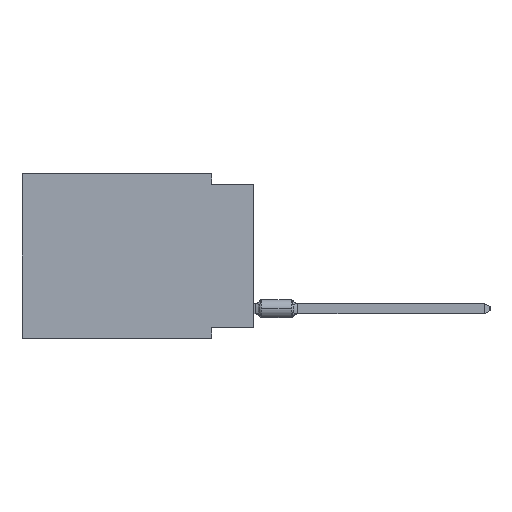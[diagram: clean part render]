
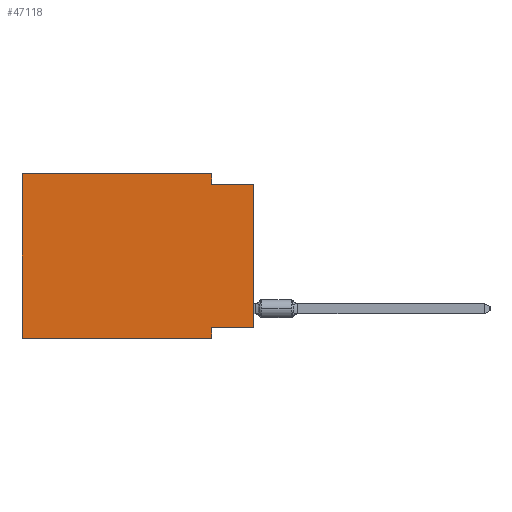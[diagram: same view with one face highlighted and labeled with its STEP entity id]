
A CAD part, left-side view. The second image highlights one B-rep face of the part: STEP entity #47118.
In plain terms, the highlighted planar face has unit normal (-1, 0, 0).
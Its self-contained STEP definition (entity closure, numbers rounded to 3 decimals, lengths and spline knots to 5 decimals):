
#24 = CARTESIAN_POINT ( 'NONE',  ( 0., 0.1, 0. ) ) ;
#1088 = ORIENTED_EDGE ( 'NONE', *, *, #34587, .F. ) ;
#1103 = CARTESIAN_POINT ( 'NONE',  ( 0., 0.1, -0.39 ) ) ;
#1213 = VERTEX_POINT ( 'NONE', #40926 ) ;
#4468 = DIRECTION ( 'NONE',  ( 0., -1., 0. ) ) ;
#4573 = CARTESIAN_POINT ( 'NONE',  ( 0., 0., -0.365 ) ) ;
#5221 = LINE ( 'NONE', #5635, #24115 ) ;
#5322 = LINE ( 'NONE', #75425, #15937 ) ;
#5595 = ORIENTED_EDGE ( 'NONE', *, *, #27650, .F. ) ;
#5635 = CARTESIAN_POINT ( 'NONE',  ( 0., 0.1, 0. ) ) ;
#7136 = VERTEX_POINT ( 'NONE', #57690 ) ;
#7254 = EDGE_CURVE ( 'NONE', #28438, #78404, #35096, .T. ) ;
#10316 = DIRECTION ( 'NONE',  ( 0., 0., -1. ) ) ;
#11436 = CARTESIAN_POINT ( 'NONE',  ( 0., 0.1, -0.365 ) ) ;
#11881 = EDGE_CURVE ( 'NONE', #24877, #19712, #24299, .T. ) ;
#14300 = DIRECTION ( 'NONE',  ( 0., -1., 0. ) ) ;
#15937 = VECTOR ( 'NONE', #4468, 39.37008 ) ;
#16603 = ORIENTED_EDGE ( 'NONE', *, *, #81407, .F. ) ;
#17672 = EDGE_CURVE ( 'NONE', #66368, #78404, #33416, .T. ) ;
#18172 = ORIENTED_EDGE ( 'NONE', *, *, #7254, .T. ) ;
#19712 = VERTEX_POINT ( 'NONE', #1103 ) ;
#21897 = ORIENTED_EDGE ( 'NONE', *, *, #11881, .F. ) ;
#24115 = VECTOR ( 'NONE', #71465, 39.37008 ) ;
#24299 = LINE ( 'NONE', #69346, #67292 ) ;
#24877 = VERTEX_POINT ( 'NONE', #11436 ) ;
#27650 = EDGE_CURVE ( 'NONE', #1213, #40995, #77255, .T. ) ;
#28190 = VECTOR ( 'NONE', #61019, 39.37008 ) ;
#28438 = VERTEX_POINT ( 'NONE', #45157 ) ;
#30576 = DIRECTION ( 'NONE',  ( 1., 0., 0. ) ) ;
#31410 = DIRECTION ( 'NONE',  ( 0., 0., -1. ) ) ;
#33416 = LINE ( 'NONE', #59343, #43852 ) ;
#34040 = EDGE_CURVE ( 'NONE', #7136, #19712, #5322, .T. ) ;
#34587 = EDGE_CURVE ( 'NONE', #40995, #66368, #5221, .T. ) ;
#35096 = LINE ( 'NONE', #40638, #28190 ) ;
#37798 = FACE_OUTER_BOUND ( 'NONE', #44434, .T. ) ;
#37963 = ORIENTED_EDGE ( 'NONE', *, *, #17672, .F. ) ;
#38252 = ORIENTED_EDGE ( 'NONE', *, *, #59425, .F. ) ;
#40638 = CARTESIAN_POINT ( 'NONE',  ( 0., 0., 0. ) ) ;
#40926 = CARTESIAN_POINT ( 'NONE',  ( 0., 0.55, 0. ) ) ;
#40995 = VERTEX_POINT ( 'NONE', #24 ) ;
#43416 = VECTOR ( 'NONE', #71725, 39.37008 ) ;
#43852 = VECTOR ( 'NONE', #14300, 39.37008 ) ;
#44434 = EDGE_LOOP ( 'NONE', ( #18172, #37963, #1088, #5595, #16603, #70477, #21897, #38252 ) ) ;
#44624 = CARTESIAN_POINT ( 'NONE',  ( 0., 0.55, 0. ) ) ;
#45157 = CARTESIAN_POINT ( 'NONE',  ( 0., 0., -0.365 ) ) ;
#46286 = AXIS2_PLACEMENT_3D ( 'NONE', #58204, #30576, #31410 ) ;
#47118 = ADVANCED_FACE ( 'NONE', ( #37798 ), #63727, .F. ) ;
#49418 = VECTOR ( 'NONE', #63760, 39.37008 ) ;
#51282 = LINE ( 'NONE', #4573, #83870 ) ;
#57378 = LINE ( 'NONE', #44624, #49418 ) ;
#57690 = CARTESIAN_POINT ( 'NONE',  ( 0., 0.55, -0.39 ) ) ;
#58204 = CARTESIAN_POINT ( 'NONE',  ( 0., 0.55, 0. ) ) ;
#59343 = CARTESIAN_POINT ( 'NONE',  ( 0., 0., -0.025 ) ) ;
#59425 = EDGE_CURVE ( 'NONE', #28438, #24877, #51282, .T. ) ;
#61019 = DIRECTION ( 'NONE',  ( 0., 0., 1. ) ) ;
#62758 = DIRECTION ( 'NONE',  ( 0., 1., 0. ) ) ;
#63727 = PLANE ( 'NONE',  #46286 ) ;
#63760 = DIRECTION ( 'NONE',  ( 0., 0., 1. ) ) ;
#64498 = CARTESIAN_POINT ( 'NONE',  ( 0., 0.55, 0. ) ) ;
#65430 = CARTESIAN_POINT ( 'NONE',  ( 0., 0., -0.025 ) ) ;
#66368 = VERTEX_POINT ( 'NONE', #72062 ) ;
#67292 = VECTOR ( 'NONE', #10316, 39.37008 ) ;
#69346 = CARTESIAN_POINT ( 'NONE',  ( 0., 0.1, -0.39 ) ) ;
#70477 = ORIENTED_EDGE ( 'NONE', *, *, #34040, .T. ) ;
#71465 = DIRECTION ( 'NONE',  ( 0., 0., -1. ) ) ;
#71725 = DIRECTION ( 'NONE',  ( 0., -1., 0. ) ) ;
#72062 = CARTESIAN_POINT ( 'NONE',  ( 0., 0.1, -0.025 ) ) ;
#75425 = CARTESIAN_POINT ( 'NONE',  ( 0., 0.55, -0.39 ) ) ;
#77255 = LINE ( 'NONE', #64498, #43416 ) ;
#78404 = VERTEX_POINT ( 'NONE', #65430 ) ;
#81407 = EDGE_CURVE ( 'NONE', #7136, #1213, #57378, .T. ) ;
#83870 = VECTOR ( 'NONE', #62758, 39.37008 ) ;
